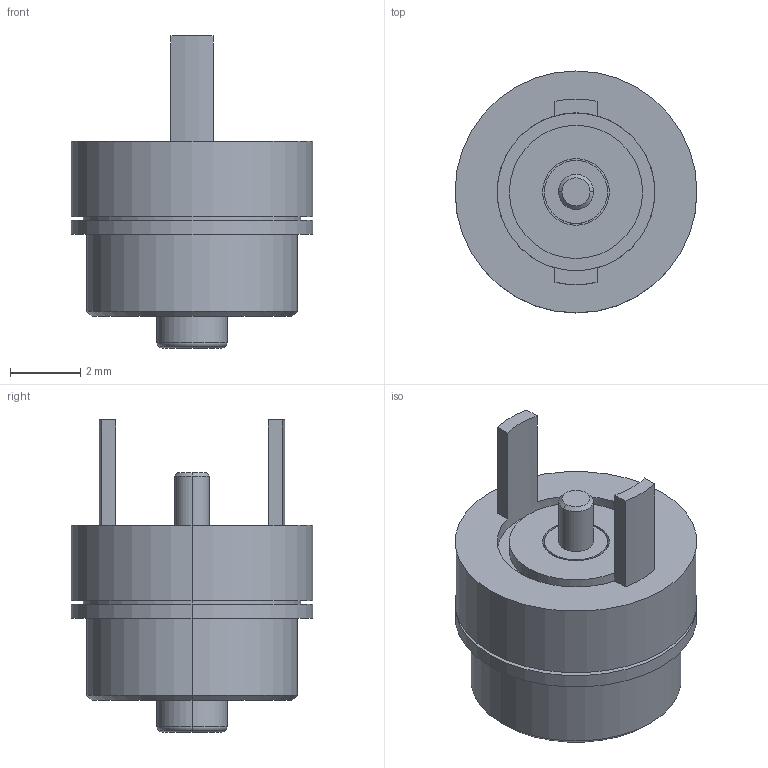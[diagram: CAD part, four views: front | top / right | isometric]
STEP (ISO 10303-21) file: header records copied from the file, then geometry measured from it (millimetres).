
FILE_DESCRIPTION (( 'STEP AP203' ), '1' );
FILE_NAME ('686-B02222030B1.STEP', '2023-02-03T17:03:51', ( 'Magnum' ), ( '' ), 'SwSTEP 2.0', 'SolidWorks 2020', '' );
FILE_SCHEMA (( 'CONFIG_CONTROL_DESIGN' ));
Length unit declared in the file: millimetre
Products named in the file (1): 686-B02222030B1
Bounding box: 6.9 x 6.9 x 8.9 mm (x, y, z)
Volume: 165.3 mm3; surface area: 434.7 mm2
Topology: 1 solids, 5 shells, 80 faces, 166 edges, 104 vertices
Faces by surface type: cylinder 38, plane 24, torus 12, cone 6
Entity records: 2243 total; most frequent: DIRECTION 436, CARTESIAN_POINT 351, ORIENTED_EDGE 332, AXIS2_PLACEMENT_3D 189, EDGE_CURVE 166, CIRCLE 108, VERTEX_POINT 104, EDGE_LOOP 96
